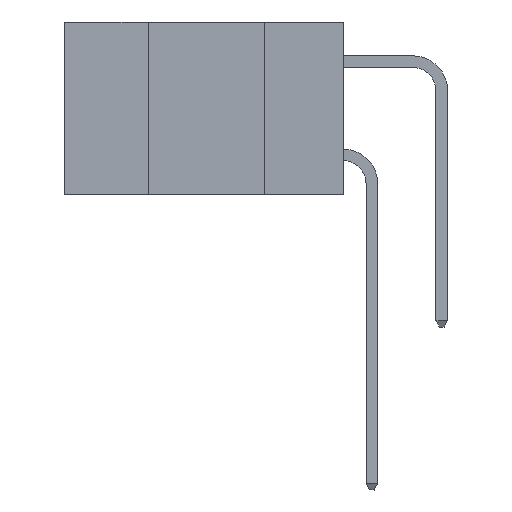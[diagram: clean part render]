
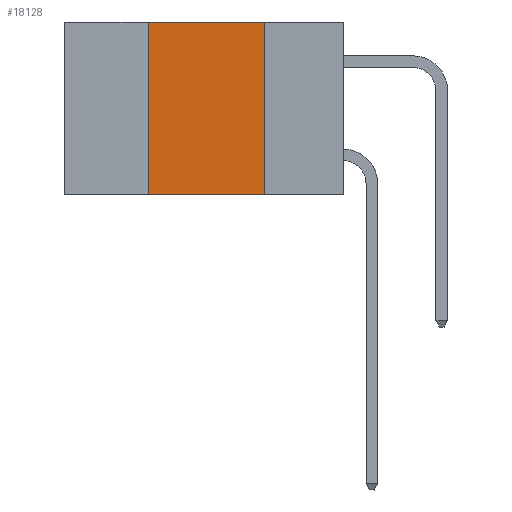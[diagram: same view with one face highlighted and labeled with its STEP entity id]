
A CAD part, left-side view. The second image highlights one B-rep face of the part: STEP entity #18128.
In plain terms, the highlighted planar face has unit normal (-1, 0, 0).
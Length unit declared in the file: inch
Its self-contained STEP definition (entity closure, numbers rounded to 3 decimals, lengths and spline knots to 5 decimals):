
#204 = EDGE_CURVE ( 'NONE', #10732, #6814, #15792, .T. ) ;
#409 = VERTEX_POINT ( 'NONE', #18459 ) ;
#569 = VERTEX_POINT ( 'NONE', #10000 ) ;
#1926 = ORIENTED_EDGE ( 'NONE', *, *, #3376, .F. ) ;
#2043 = LINE ( 'NONE', #14492, #5496 ) ;
#2426 = CARTESIAN_POINT ( 'NONE',  ( 0., 0.6, 0. ) ) ;
#2689 = ORIENTED_EDGE ( 'NONE', *, *, #16515, .F. ) ;
#3376 = EDGE_CURVE ( 'NONE', #569, #409, #2043, .T. ) ;
#3901 = DIRECTION ( 'NONE',  ( 0., 0., -1. ) ) ;
#5367 = CARTESIAN_POINT ( 'NONE',  ( 0., 0.17, -0.37 ) ) ;
#5496 = VECTOR ( 'NONE', #9172, 39.37008 ) ;
#6814 = VERTEX_POINT ( 'NONE', #5367 ) ;
#7884 = DIRECTION ( 'NONE',  ( 0., 0., -1. ) ) ;
#8187 = PLANE ( 'NONE',  #18843 ) ;
#8369 = ORIENTED_EDGE ( 'NONE', *, *, #17964, .F. ) ;
#8388 = CARTESIAN_POINT ( 'NONE',  ( 0., 0.42, 0. ) ) ;
#8535 = LINE ( 'NONE', #8388, #12005 ) ;
#9172 = DIRECTION ( 'NONE',  ( 0., -1., 0. ) ) ;
#9513 = EDGE_LOOP ( 'NONE', ( #8369, #1926, #2689, #9675 ) ) ;
#9675 = ORIENTED_EDGE ( 'NONE', *, *, #204, .T. ) ;
#10000 = CARTESIAN_POINT ( 'NONE',  ( 0., 0.42, 0. ) ) ;
#10732 = VERTEX_POINT ( 'NONE', #13079 ) ;
#11365 = DIRECTION ( 'NONE',  ( 0., 0., 1. ) ) ;
#12005 = VECTOR ( 'NONE', #11365, 39.37008 ) ;
#12457 = VECTOR ( 'NONE', #13903, 39.37008 ) ;
#12625 = DIRECTION ( 'NONE',  ( 1., 0., 0. ) ) ;
#13079 = CARTESIAN_POINT ( 'NONE',  ( 0., 0.42, -0.37 ) ) ;
#13903 = DIRECTION ( 'NONE',  ( 0., -1., 0. ) ) ;
#14492 = CARTESIAN_POINT ( 'NONE',  ( 0., 0.6, 0. ) ) ;
#15089 = VECTOR ( 'NONE', #7884, 39.37008 ) ;
#15121 = CARTESIAN_POINT ( 'NONE',  ( 0., 0.17, 0. ) ) ;
#15792 = LINE ( 'NONE', #18592, #12457 ) ;
#16515 = EDGE_CURVE ( 'NONE', #10732, #569, #8535, .T. ) ;
#16666 = FACE_OUTER_BOUND ( 'NONE', #9513, .T. ) ;
#17964 = EDGE_CURVE ( 'NONE', #409, #6814, #18881, .T. ) ;
#18128 = ADVANCED_FACE ( 'NONE', ( #16666 ), #8187, .F. ) ;
#18459 = CARTESIAN_POINT ( 'NONE',  ( 0., 0.17, 0. ) ) ;
#18592 = CARTESIAN_POINT ( 'NONE',  ( 0., 0.6, -0.37 ) ) ;
#18843 = AXIS2_PLACEMENT_3D ( 'NONE', #2426, #12625, #3901 ) ;
#18881 = LINE ( 'NONE', #15121, #15089 ) ;
